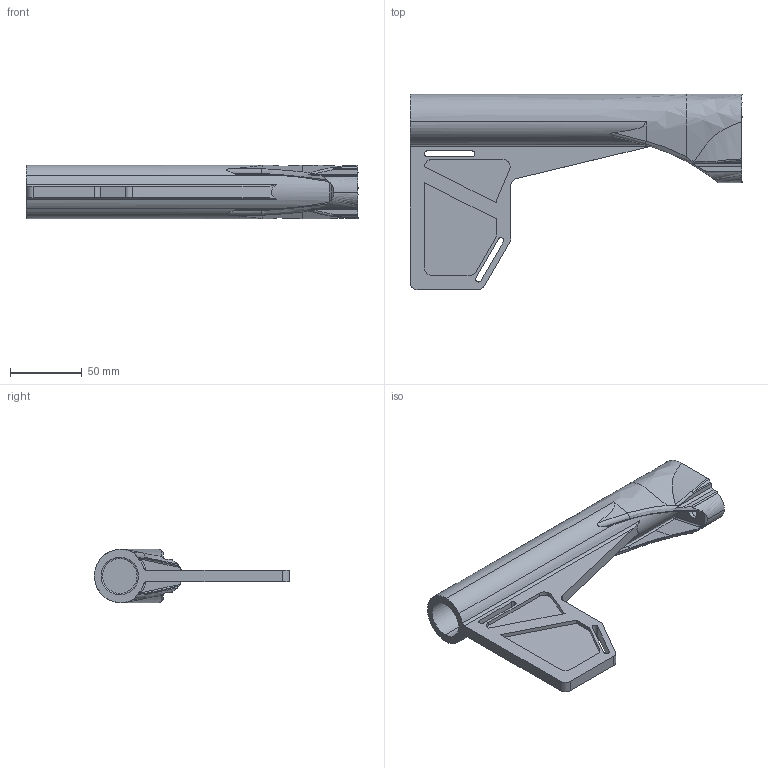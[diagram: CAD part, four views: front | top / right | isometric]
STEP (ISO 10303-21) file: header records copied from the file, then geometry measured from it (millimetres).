
FILE_DESCRIPTION (( 'STEP AP203' ), '1' );
FILE_NAME ('mbbi_monopoly_rear_brace_v1.0.STEP', '2022-06-11T20:02:21', ( '' ), ( '' ), 'SwSTEP 2.0', 'SolidWorks 2021', '' );
FILE_SCHEMA (( 'CONFIG_CONTROL_DESIGN' ));
Length unit declared in the file: millimetre
Products named in the file (1): mbbi_monopoly_rear_brace_v1.0
Bounding box: 230.77 x 135.64 x 37.13 mm (x, y, z)
Volume: 167330.8 mm3; surface area: 73232 mm2
Topology: 1 solids, 1 shells, 154 faces, 418 edges, 273 vertices
Faces by surface type: plane 68, cylinder 46, bspline 29, torus 7, sphere 4
Entity records: 6957 total; most frequent: CARTESIAN_POINT 3240, ORIENTED_EDGE 828, DIRECTION 656, EDGE_CURVE 414, VERTEX_POINT 271, AXIS2_PLACEMENT_3D 227, VECTOR 202, LINE 202
